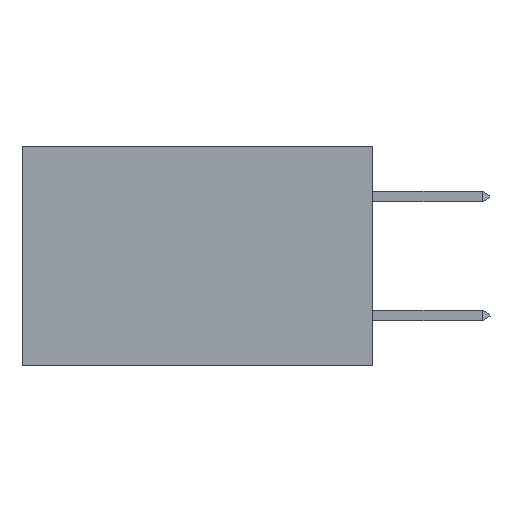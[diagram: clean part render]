
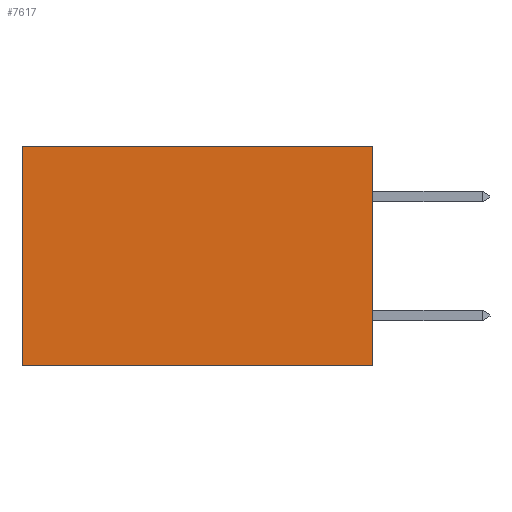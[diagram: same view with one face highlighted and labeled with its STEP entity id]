
A CAD part, left-side view. The second image highlights one B-rep face of the part: STEP entity #7617.
In plain terms, the highlighted planar face has unit normal (-1, 0, 0).
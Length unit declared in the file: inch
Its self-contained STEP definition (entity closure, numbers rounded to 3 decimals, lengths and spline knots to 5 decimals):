
#2 = VECTOR ( 'NONE', #6634, 39.37008 ) ;
#368 = EDGE_CURVE ( 'NONE', #8010, #6039, #7380, .T. ) ;
#513 = ORIENTED_EDGE ( 'NONE', *, *, #11804, .T. ) ;
#564 = LINE ( 'NONE', #5701, #2 ) ;
#865 = EDGE_CURVE ( 'NONE', #1751, #9927, #10715, .T. ) ;
#898 = CARTESIAN_POINT ( 'NONE',  ( 0.277, 0., 0. ) ) ;
#949 = DIRECTION ( 'NONE',  ( 0., 1., 0. ) ) ;
#960 = ORIENTED_EDGE ( 'NONE', *, *, #368, .T. ) ;
#1751 = VERTEX_POINT ( 'NONE', #3337 ) ;
#2000 = AXIS2_PLACEMENT_3D ( 'NONE', #2745, #9201, #3689 ) ;
#2345 = CARTESIAN_POINT ( 'NONE',  ( 0.277, 0.59, -0.37 ) ) ;
#2745 = CARTESIAN_POINT ( 'NONE',  ( 0.277, 0., -0.37 ) ) ;
#2830 = CARTESIAN_POINT ( 'NONE',  ( 0.277, 0.59, -0.37 ) ) ;
#3337 = CARTESIAN_POINT ( 'NONE',  ( 0.277, 0., -0.37 ) ) ;
#3689 = DIRECTION ( 'NONE',  ( 0., 0., -1. ) ) ;
#5304 = FACE_OUTER_BOUND ( 'NONE', #6258, .T. ) ;
#5701 = CARTESIAN_POINT ( 'NONE',  ( 0.277, 0., -0.37 ) ) ;
#6039 = VERTEX_POINT ( 'NONE', #8148 ) ;
#6258 = EDGE_LOOP ( 'NONE', ( #513, #10493, #6672, #960 ) ) ;
#6484 = PLANE ( 'NONE',  #2000 ) ;
#6634 = DIRECTION ( 'NONE',  ( 0., 0., -1. ) ) ;
#6672 = ORIENTED_EDGE ( 'NONE', *, *, #11295, .F. ) ;
#7153 = DIRECTION ( 'NONE',  ( 0., 1., 0. ) ) ;
#7380 = LINE ( 'NONE', #898, #9186 ) ;
#7617 = ADVANCED_FACE ( 'NONE', ( #5304 ), #6484, .F. ) ;
#8010 = VERTEX_POINT ( 'NONE', #11506 ) ;
#8148 = CARTESIAN_POINT ( 'NONE',  ( 0.277, 0.59, 0. ) ) ;
#8360 = VECTOR ( 'NONE', #7153, 39.37008 ) ;
#8684 = VECTOR ( 'NONE', #10167, 39.37008 ) ;
#8949 = LINE ( 'NONE', #2830, #8684 ) ;
#9141 = CARTESIAN_POINT ( 'NONE',  ( 0.277, 0., -0.37 ) ) ;
#9186 = VECTOR ( 'NONE', #949, 39.37008 ) ;
#9201 = DIRECTION ( 'NONE',  ( 1., 0., 0. ) ) ;
#9927 = VERTEX_POINT ( 'NONE', #2345 ) ;
#10167 = DIRECTION ( 'NONE',  ( 0., 0., -1. ) ) ;
#10493 = ORIENTED_EDGE ( 'NONE', *, *, #865, .F. ) ;
#10715 = LINE ( 'NONE', #9141, #8360 ) ;
#11295 = EDGE_CURVE ( 'NONE', #8010, #1751, #564, .T. ) ;
#11506 = CARTESIAN_POINT ( 'NONE',  ( 0.277, 0., 0. ) ) ;
#11804 = EDGE_CURVE ( 'NONE', #6039, #9927, #8949, .T. ) ;
